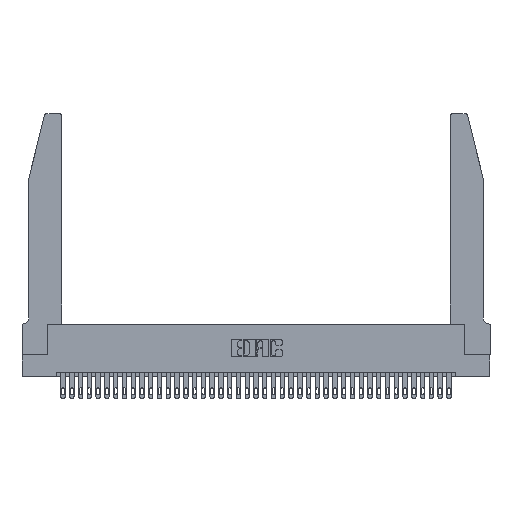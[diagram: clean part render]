
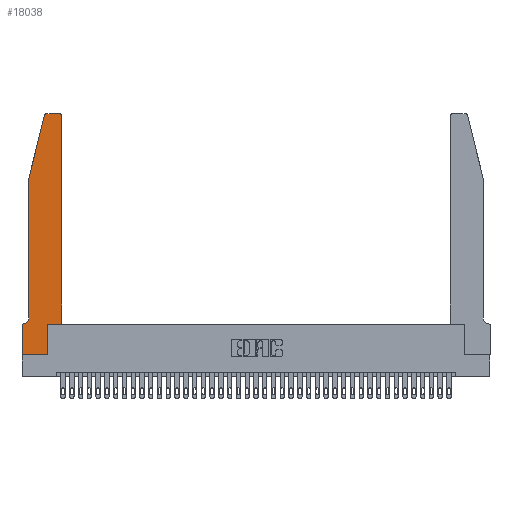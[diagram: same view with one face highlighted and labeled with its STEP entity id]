
A CAD part, top view. The second image highlights one B-rep face of the part: STEP entity #18038.
In plain terms, the highlighted planar face has unit normal (0, 0, 1).
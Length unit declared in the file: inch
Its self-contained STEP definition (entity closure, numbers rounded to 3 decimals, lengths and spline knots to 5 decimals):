
#449 = AXIS2_PLACEMENT_3D ( 'NONE', #5089, #16822, #1879 ) ;
#1198 = CARTESIAN_POINT ( 'NONE',  ( 0.0755, 2., 0.37 ) ) ;
#1529 = LINE ( 'NONE', #5362, #30738 ) ;
#1879 = DIRECTION ( 'NONE',  ( 1., 0., 0. ) ) ;
#1994 = DIRECTION ( 'NONE',  ( 0., 0., 1. ) ) ;
#2298 = VECTOR ( 'NONE', #37706, 39.37008 ) ;
#2770 = EDGE_CURVE ( 'NONE', #24853, #38152, #17281, .T. ) ;
#3062 = VERTEX_POINT ( 'NONE', #9169 ) ;
#3669 = VECTOR ( 'NONE', #33656, 39.37008 ) ;
#4064 = ORIENTED_EDGE ( 'NONE', *, *, #19218, .T. ) ;
#4258 = VERTEX_POINT ( 'NONE', #8325 ) ;
#4348 = VERTEX_POINT ( 'NONE', #13013 ) ;
#4953 = PLANE ( 'NONE',  #21506 ) ;
#5089 = CARTESIAN_POINT ( 'NONE',  ( 0.284, 2.72, 0.37 ) ) ;
#5362 = CARTESIAN_POINT ( 'NONE',  ( 0.2605, 2.75, 0.37 ) ) ;
#5500 = VECTOR ( 'NONE', #31100, 39.37008 ) ;
#5615 = EDGE_LOOP ( 'NONE', ( #20601, #8336, #33334, #38421, #13216, #37086, #15315, #4064, #7584, #30116, #24310, #17219 ) ) ;
#5824 = DIRECTION ( 'NONE',  ( -0.239, -0.971, 0. ) ) ;
#5845 = VECTOR ( 'NONE', #5824, 39.37008 ) ;
#5934 = EDGE_CURVE ( 'NONE', #4348, #22476, #24973, .T. ) ;
#6962 = CARTESIAN_POINT ( 'NONE',  ( 0.0055, 0.35, 0.37 ) ) ;
#7584 = ORIENTED_EDGE ( 'NONE', *, *, #5934, .T. ) ;
#7720 = EDGE_CURVE ( 'NONE', #38178, #20717, #17270, .T. ) ;
#8257 = CARTESIAN_POINT ( 'NONE',  ( 0., 0.35, 0.37 ) ) ;
#8272 = DIRECTION ( 'NONE',  ( -1., 0., 0. ) ) ;
#8325 = CARTESIAN_POINT ( 'NONE',  ( 0.4205, 2.75, 0.37 ) ) ;
#8336 = ORIENTED_EDGE ( 'NONE', *, *, #29312, .T. ) ;
#8796 = DIRECTION ( 'NONE',  ( 0., 0., 1. ) ) ;
#8926 = DIRECTION ( 'NONE',  ( 1., 0., 0. ) ) ;
#9169 = CARTESIAN_POINT ( 'NONE',  ( 0.284, 2.75, 0.37 ) ) ;
#10016 = CARTESIAN_POINT ( 'NONE',  ( 0., 0., 0.37 ) ) ;
#10023 = VECTOR ( 'NONE', #23317, 39.37008 ) ;
#11069 = EDGE_CURVE ( 'NONE', #15266, #17552, #30289, .T. ) ;
#11508 = VERTEX_POINT ( 'NONE', #31685 ) ;
#11550 = VECTOR ( 'NONE', #27709, 39.37008 ) ;
#12433 = AXIS2_PLACEMENT_3D ( 'NONE', #28079, #8796, #8926 ) ;
#12800 = LINE ( 'NONE', #10016, #13883 ) ;
#13013 = CARTESIAN_POINT ( 'NONE',  ( 0.2865, 0., 0.37 ) ) ;
#13216 = ORIENTED_EDGE ( 'NONE', *, *, #2770, .T. ) ;
#13228 = LINE ( 'NONE', #26056, #2298 ) ;
#13711 = CARTESIAN_POINT ( 'NONE',  ( 0.4505, 0.35, 0.37 ) ) ;
#13883 = VECTOR ( 'NONE', #19235, 39.37008 ) ;
#15071 = EDGE_CURVE ( 'NONE', #17552, #4258, #36610, .T. ) ;
#15266 = VERTEX_POINT ( 'NONE', #13711 ) ;
#15315 = ORIENTED_EDGE ( 'NONE', *, *, #34484, .T. ) ;
#15433 = CARTESIAN_POINT ( 'NONE',  ( 0., 0., 0.37 ) ) ;
#15580 = EDGE_CURVE ( 'NONE', #20717, #24853, #29901, .T. ) ;
#16477 = DIRECTION ( 'NONE',  ( 0., 1., 0. ) ) ;
#16822 = DIRECTION ( 'NONE',  ( 0., 0., 1. ) ) ;
#17219 = ORIENTED_EDGE ( 'NONE', *, *, #15071, .T. ) ;
#17270 = LINE ( 'NONE', #1198, #5845 ) ;
#17281 = CIRCLE ( 'NONE', #33985, 0.07 ) ;
#17512 = CARTESIAN_POINT ( 'NONE',  ( 0.0755, 2., 0.37 ) ) ;
#17552 = VERTEX_POINT ( 'NONE', #21065 ) ;
#18038 = ADVANCED_FACE ( 'NONE', ( #35334 ), #4953, .T. ) ;
#18061 = CARTESIAN_POINT ( 'NONE',  ( 0.2865, 0.35, 0.37 ) ) ;
#18396 = EDGE_CURVE ( 'NONE', #22476, #15266, #13228, .T. ) ;
#19218 = EDGE_CURVE ( 'NONE', #36125, #4348, #19895, .T. ) ;
#19235 = DIRECTION ( 'NONE',  ( 0., -1., 0. ) ) ;
#19847 = CARTESIAN_POINT ( 'NONE',  ( 0.0055, 0.42, 0.37 ) ) ;
#19895 = LINE ( 'NONE', #27382, #3669 ) ;
#20085 = LINE ( 'NONE', #20092, #10023 ) ;
#20092 = CARTESIAN_POINT ( 'NONE',  ( 0.0755, 0.35, 0.37 ) ) ;
#20601 = ORIENTED_EDGE ( 'NONE', *, *, #32930, .T. ) ;
#20717 = VERTEX_POINT ( 'NONE', #17512 ) ;
#21065 = CARTESIAN_POINT ( 'NONE',  ( 0.4505, 2.72, 0.37 ) ) ;
#21506 = AXIS2_PLACEMENT_3D ( 'NONE', #8257, #1994, #26323 ) ;
#22241 = CARTESIAN_POINT ( 'NONE',  ( 0.0755, 2., 0.37 ) ) ;
#22476 = VERTEX_POINT ( 'NONE', #18061 ) ;
#23317 = DIRECTION ( 'NONE',  ( -1., 0., 0. ) ) ;
#24310 = ORIENTED_EDGE ( 'NONE', *, *, #11069, .T. ) ;
#24853 = VERTEX_POINT ( 'NONE', #26212 ) ;
#24973 = LINE ( 'NONE', #36144, #11550 ) ;
#26056 = CARTESIAN_POINT ( 'NONE',  ( 0.4505, 0.35, 0.37 ) ) ;
#26212 = CARTESIAN_POINT ( 'NONE',  ( 0.0755, 0.42, 0.37 ) ) ;
#26323 = DIRECTION ( 'NONE',  ( 1., 0., 0. ) ) ;
#26579 = CIRCLE ( 'NONE', #449, 0.03 ) ;
#27382 = CARTESIAN_POINT ( 'NONE',  ( 0., 0., 0.37 ) ) ;
#27709 = DIRECTION ( 'NONE',  ( 0., 1., 0. ) ) ;
#28079 = CARTESIAN_POINT ( 'NONE',  ( 0.4205, 2.72, 0.37 ) ) ;
#28375 = EDGE_CURVE ( 'NONE', #38152, #11508, #20085, .T. ) ;
#29312 = EDGE_CURVE ( 'NONE', #3062, #38178, #26579, .T. ) ;
#29901 = LINE ( 'NONE', #22241, #5500 ) ;
#30116 = ORIENTED_EDGE ( 'NONE', *, *, #18396, .T. ) ;
#30289 = LINE ( 'NONE', #31768, #34558 ) ;
#30738 = VECTOR ( 'NONE', #8272, 39.37008 ) ;
#31100 = DIRECTION ( 'NONE',  ( 0., -1., 0. ) ) ;
#31544 = DIRECTION ( 'NONE',  ( -1., 0., 0. ) ) ;
#31685 = CARTESIAN_POINT ( 'NONE',  ( 0., 0.35, 0.37 ) ) ;
#31768 = CARTESIAN_POINT ( 'NONE',  ( 0.4505, 0.35, 0.37 ) ) ;
#31813 = DIRECTION ( 'NONE',  ( 0., 0., -1. ) ) ;
#32930 = EDGE_CURVE ( 'NONE', #4258, #3062, #1529, .T. ) ;
#33334 = ORIENTED_EDGE ( 'NONE', *, *, #7720, .T. ) ;
#33656 = DIRECTION ( 'NONE',  ( 1., 0., 0. ) ) ;
#33985 = AXIS2_PLACEMENT_3D ( 'NONE', #19847, #31813, #31544 ) ;
#34484 = EDGE_CURVE ( 'NONE', #11508, #36125, #12800, .T. ) ;
#34558 = VECTOR ( 'NONE', #16477, 39.37008 ) ;
#35334 = FACE_OUTER_BOUND ( 'NONE', #5615, .T. ) ;
#36125 = VERTEX_POINT ( 'NONE', #15433 ) ;
#36144 = CARTESIAN_POINT ( 'NONE',  ( 0.2865, 0.35, 0.37 ) ) ;
#36610 = CIRCLE ( 'NONE', #12433, 0.03 ) ;
#37086 = ORIENTED_EDGE ( 'NONE', *, *, #28375, .T. ) ;
#37475 = CARTESIAN_POINT ( 'NONE',  ( 0.25487, 2.72718, 0.37 ) ) ;
#37706 = DIRECTION ( 'NONE',  ( 1., 0., 0. ) ) ;
#38152 = VERTEX_POINT ( 'NONE', #6962 ) ;
#38178 = VERTEX_POINT ( 'NONE', #37475 ) ;
#38421 = ORIENTED_EDGE ( 'NONE', *, *, #15580, .T. ) ;
